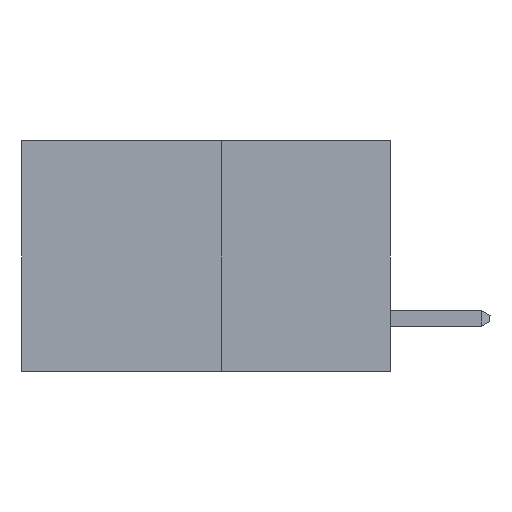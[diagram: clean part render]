
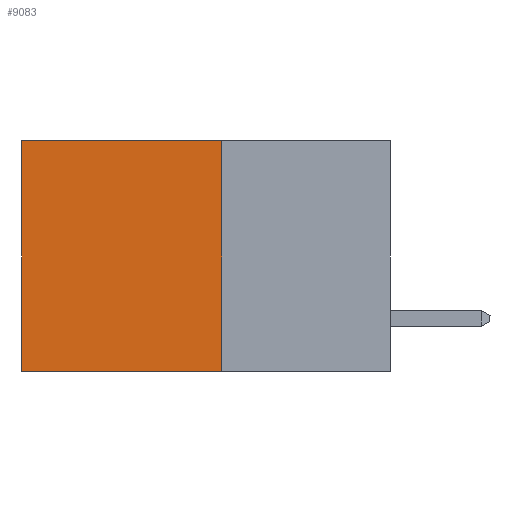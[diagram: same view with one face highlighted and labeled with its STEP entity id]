
A CAD part, left-side view. The second image highlights one B-rep face of the part: STEP entity #9083.
In plain terms, the highlighted planar face has unit normal (-1, 0, 0).
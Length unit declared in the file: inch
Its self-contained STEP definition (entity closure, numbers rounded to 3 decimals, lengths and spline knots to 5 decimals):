
#350 = EDGE_LOOP ( 'NONE', ( #14222, #11246, #13806, #1553 ) ) ;
#1150 = CARTESIAN_POINT ( 'NONE',  ( 0.277, 0.27, -0.37 ) ) ;
#1231 = LINE ( 'NONE', #8820, #8193 ) ;
#1553 = ORIENTED_EDGE ( 'NONE', *, *, #4153, .T. ) ;
#1943 = EDGE_CURVE ( 'NONE', #12928, #15521, #10833, .T. ) ;
#2056 = CARTESIAN_POINT ( 'NONE',  ( 0.277, 0.27, -0.37 ) ) ;
#2665 = VECTOR ( 'NONE', #10097, 39.37008 ) ;
#2705 = LINE ( 'NONE', #4594, #6004 ) ;
#3568 = DIRECTION ( 'NONE',  ( 0., 1., 0. ) ) ;
#4153 = EDGE_CURVE ( 'NONE', #12928, #6756, #2705, .T. ) ;
#4284 = AXIS2_PLACEMENT_3D ( 'NONE', #11869, #6526, #15657 ) ;
#4594 = CARTESIAN_POINT ( 'NONE',  ( 0.277, 0.27, 0. ) ) ;
#5739 = VECTOR ( 'NONE', #12907, 39.37008 ) ;
#6004 = VECTOR ( 'NONE', #3568, 39.37008 ) ;
#6526 = DIRECTION ( 'NONE',  ( 1., 0., 0. ) ) ;
#6744 = CARTESIAN_POINT ( 'NONE',  ( 0.277, 0.27, -0.37 ) ) ;
#6756 = VERTEX_POINT ( 'NONE', #14631 ) ;
#8193 = VECTOR ( 'NONE', #11500, 39.37008 ) ;
#8229 = EDGE_CURVE ( 'NONE', #6756, #9088, #1231, .T. ) ;
#8820 = CARTESIAN_POINT ( 'NONE',  ( 0.277, 0.59, -0.37 ) ) ;
#9083 = ADVANCED_FACE ( 'NONE', ( #17202 ), #14382, .F. ) ;
#9088 = VERTEX_POINT ( 'NONE', #10611 ) ;
#10097 = DIRECTION ( 'NONE',  ( 0., 0., -1. ) ) ;
#10611 = CARTESIAN_POINT ( 'NONE',  ( 0.277, 0.59, -0.37 ) ) ;
#10833 = LINE ( 'NONE', #6744, #2665 ) ;
#11246 = ORIENTED_EDGE ( 'NONE', *, *, #13660, .F. ) ;
#11500 = DIRECTION ( 'NONE',  ( 0., 0., -1. ) ) ;
#11869 = CARTESIAN_POINT ( 'NONE',  ( 0.277, 0.27, -0.37 ) ) ;
#12907 = DIRECTION ( 'NONE',  ( 0., 1., 0. ) ) ;
#12928 = VERTEX_POINT ( 'NONE', #15232 ) ;
#13660 = EDGE_CURVE ( 'NONE', #15521, #9088, #16631, .T. ) ;
#13806 = ORIENTED_EDGE ( 'NONE', *, *, #1943, .F. ) ;
#14222 = ORIENTED_EDGE ( 'NONE', *, *, #8229, .T. ) ;
#14382 = PLANE ( 'NONE',  #4284 ) ;
#14631 = CARTESIAN_POINT ( 'NONE',  ( 0.277, 0.59, 0. ) ) ;
#15232 = CARTESIAN_POINT ( 'NONE',  ( 0.277, 0.27, 0. ) ) ;
#15521 = VERTEX_POINT ( 'NONE', #1150 ) ;
#15657 = DIRECTION ( 'NONE',  ( 0., 0., -1. ) ) ;
#16631 = LINE ( 'NONE', #2056, #5739 ) ;
#17202 = FACE_OUTER_BOUND ( 'NONE', #350, .T. ) ;
